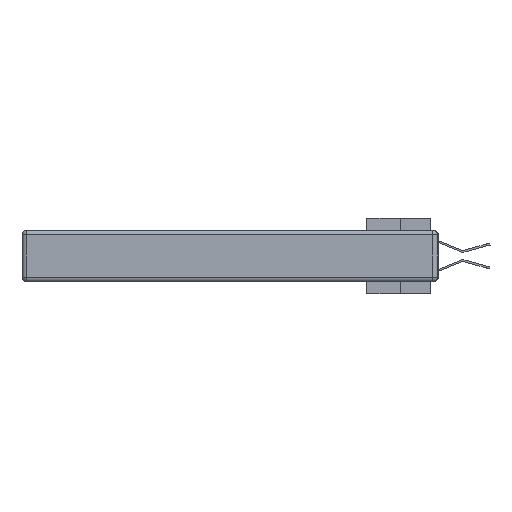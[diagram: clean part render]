
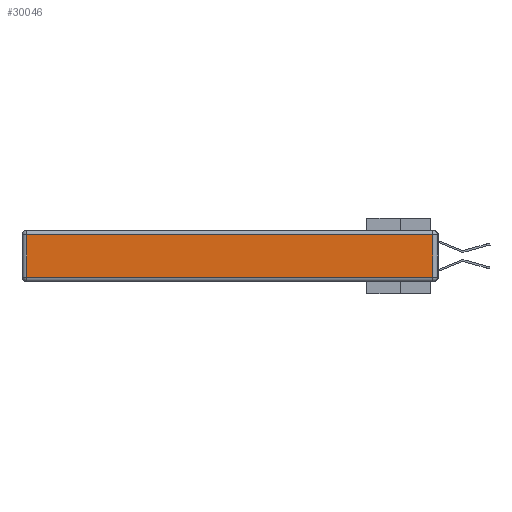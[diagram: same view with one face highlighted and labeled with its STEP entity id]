
A CAD part, left-side view. The second image highlights one B-rep face of the part: STEP entity #30046.
In plain terms, the highlighted planar face has unit normal (-1, 0, 0).
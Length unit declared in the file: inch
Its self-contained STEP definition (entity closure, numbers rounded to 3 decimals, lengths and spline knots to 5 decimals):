
#106 = CARTESIAN_POINT ( 'NONE',  ( 0., 0.03, -0.343 ) ) ;
#1074 = EDGE_CURVE ( 'NONE', #7926, #8898, #7246, .T. ) ;
#2414 = CARTESIAN_POINT ( 'NONE',  ( 0., 0., -0.313 ) ) ;
#4183 = DIRECTION ( 'NONE',  ( 0., 0., -1. ) ) ;
#6241 = DIRECTION ( 'NONE',  ( -1., 0., 0. ) ) ;
#7246 = LINE ( 'NONE', #2414, #31364 ) ;
#7488 = DIRECTION ( 'NONE',  ( 0., 0., 1. ) ) ;
#7926 = VERTEX_POINT ( 'NONE', #13593 ) ;
#7927 = EDGE_CURVE ( 'NONE', #8898, #8826, #21067, .T. ) ;
#8358 = ORIENTED_EDGE ( 'NONE', *, *, #13838, .T. ) ;
#8644 = PLANE ( 'NONE',  #17224 ) ;
#8805 = CARTESIAN_POINT ( 'NONE',  ( 0., 0., -0.343 ) ) ;
#8826 = VERTEX_POINT ( 'NONE', #19515 ) ;
#8898 = VERTEX_POINT ( 'NONE', #17076 ) ;
#9060 = VECTOR ( 'NONE', #29753, 39.37008 ) ;
#9447 = LINE ( 'NONE', #19302, #9060 ) ;
#9784 = VECTOR ( 'NONE', #4183, 39.37008 ) ;
#12209 = DIRECTION ( 'NONE',  ( 0., -1., 0. ) ) ;
#13593 = CARTESIAN_POINT ( 'NONE',  ( 0., 2.72, -0.313 ) ) ;
#13838 = EDGE_CURVE ( 'NONE', #8826, #17841, #9447, .T. ) ;
#17076 = CARTESIAN_POINT ( 'NONE',  ( 0., 0.03, -0.313 ) ) ;
#17224 = AXIS2_PLACEMENT_3D ( 'NONE', #8805, #6241, #20413 ) ;
#17841 = VERTEX_POINT ( 'NONE', #20559 ) ;
#19302 = CARTESIAN_POINT ( 'NONE',  ( 0., 2.75, -0.03 ) ) ;
#19515 = CARTESIAN_POINT ( 'NONE',  ( 0., 0.03, -0.03 ) ) ;
#20413 = DIRECTION ( 'NONE',  ( 0., 0., 1. ) ) ;
#20559 = CARTESIAN_POINT ( 'NONE',  ( 0., 2.72, -0.03 ) ) ;
#20784 = CARTESIAN_POINT ( 'NONE',  ( 0., 2.72, -0.343 ) ) ;
#21067 = LINE ( 'NONE', #106, #25811 ) ;
#21540 = ORIENTED_EDGE ( 'NONE', *, *, #24778, .T. ) ;
#24215 = ORIENTED_EDGE ( 'NONE', *, *, #7927, .T. ) ;
#24778 = EDGE_CURVE ( 'NONE', #17841, #7926, #30931, .T. ) ;
#25811 = VECTOR ( 'NONE', #7488, 39.37008 ) ;
#26571 = ORIENTED_EDGE ( 'NONE', *, *, #1074, .T. ) ;
#27846 = FACE_OUTER_BOUND ( 'NONE', #30256, .T. ) ;
#29753 = DIRECTION ( 'NONE',  ( 0., 1., 0. ) ) ;
#30046 = ADVANCED_FACE ( 'NONE', ( #27846 ), #8644, .T. ) ;
#30256 = EDGE_LOOP ( 'NONE', ( #26571, #24215, #8358, #21540 ) ) ;
#30931 = LINE ( 'NONE', #20784, #9784 ) ;
#31364 = VECTOR ( 'NONE', #12209, 39.37008 ) ;
